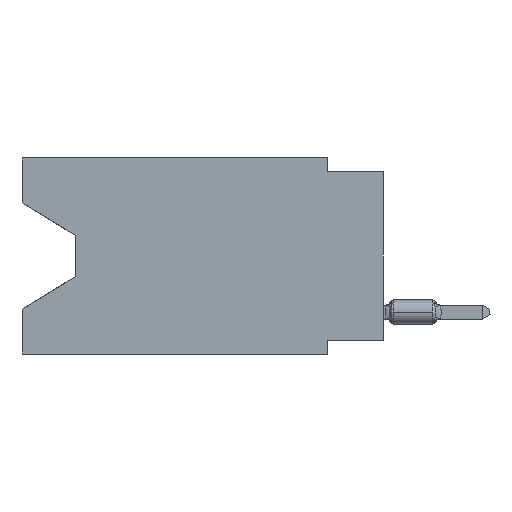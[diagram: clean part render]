
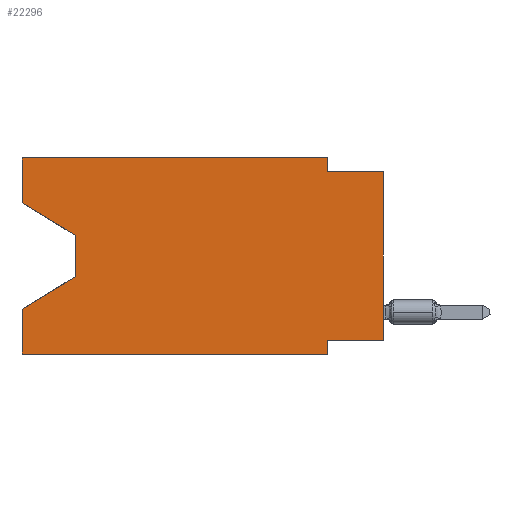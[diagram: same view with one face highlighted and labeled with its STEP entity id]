
A CAD part, left-side view. The second image highlights one B-rep face of the part: STEP entity #22296.
In plain terms, the highlighted planar face has unit normal (-1, 0, 0).
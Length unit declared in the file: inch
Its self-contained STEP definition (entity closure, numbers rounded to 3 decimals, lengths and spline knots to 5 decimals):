
#964 = CARTESIAN_POINT ( 'NONE',  ( 0., 0.645, 0. ) ) ;
#1428 = EDGE_CURVE ( 'NONE', #8827, #56739, #14687, .T. ) ;
#2313 = DIRECTION ( 'NONE',  ( 0., -1., 0. ) ) ;
#3526 = VERTEX_POINT ( 'NONE', #34012 ) ;
#4070 = CARTESIAN_POINT ( 'NONE',  ( 0., 0.55, -0.212 ) ) ;
#4557 = ORIENTED_EDGE ( 'NONE', *, *, #1428, .F. ) ;
#4574 = VERTEX_POINT ( 'NONE', #27284 ) ;
#5607 = VERTEX_POINT ( 'NONE', #44776 ) ;
#6593 = VECTOR ( 'NONE', #7825, 39.37008 ) ;
#6645 = DIRECTION ( 'NONE',  ( 0., 0., 1. ) ) ;
#7280 = CARTESIAN_POINT ( 'NONE',  ( 0., 0., -0.325 ) ) ;
#7825 = DIRECTION ( 'NONE',  ( 0., 0.855, -0.519 ) ) ;
#8555 = DIRECTION ( 'NONE',  ( 0., 0., 1. ) ) ;
#8827 = VERTEX_POINT ( 'NONE', #23724 ) ;
#10400 = EDGE_CURVE ( 'NONE', #5607, #15619, #30885, .T. ) ;
#10665 = LINE ( 'NONE', #19265, #46257 ) ;
#10930 = CARTESIAN_POINT ( 'NONE',  ( 0., 0.645, 0. ) ) ;
#11204 = FACE_OUTER_BOUND ( 'NONE', #55167, .T. ) ;
#11946 = ORIENTED_EDGE ( 'NONE', *, *, #47086, .F. ) ;
#12207 = CARTESIAN_POINT ( 'NONE',  ( 0., 0.645, -0.08025 ) ) ;
#12416 = VERTEX_POINT ( 'NONE', #50872 ) ;
#12481 = EDGE_CURVE ( 'NONE', #49396, #56739, #15259, .T. ) ;
#12950 = CARTESIAN_POINT ( 'NONE',  ( 0., 0.1, -0.35 ) ) ;
#13153 = LINE ( 'NONE', #21472, #21382 ) ;
#13313 = VECTOR ( 'NONE', #46690, 39.37008 ) ;
#13535 = CARTESIAN_POINT ( 'NONE',  ( 0., 0., -0.025 ) ) ;
#14687 = LINE ( 'NONE', #23007, #40045 ) ;
#15259 = LINE ( 'NONE', #29590, #23936 ) ;
#15532 = DIRECTION ( 'NONE',  ( 0., 0., -1. ) ) ;
#15619 = VERTEX_POINT ( 'NONE', #42896 ) ;
#15879 = VERTEX_POINT ( 'NONE', #16654 ) ;
#15883 = CARTESIAN_POINT ( 'NONE',  ( 0., 0.645, -0.26975 ) ) ;
#16369 = ORIENTED_EDGE ( 'NONE', *, *, #50506, .T. ) ;
#16379 = ORIENTED_EDGE ( 'NONE', *, *, #12481, .T. ) ;
#16654 = CARTESIAN_POINT ( 'NONE',  ( 0., 0.55, -0.212 ) ) ;
#16990 = LINE ( 'NONE', #46628, #45566 ) ;
#17529 = ORIENTED_EDGE ( 'NONE', *, *, #39760, .F. ) ;
#18486 = DIRECTION ( 'NONE',  ( 0., -1., 0. ) ) ;
#18595 = ORIENTED_EDGE ( 'NONE', *, *, #30845, .F. ) ;
#19265 = CARTESIAN_POINT ( 'NONE',  ( 0., 0.55, -0.138 ) ) ;
#20377 = CARTESIAN_POINT ( 'NONE',  ( 0., 0., -0.325 ) ) ;
#20718 = VERTEX_POINT ( 'NONE', #33764 ) ;
#21382 = VECTOR ( 'NONE', #8555, 39.37008 ) ;
#21472 = CARTESIAN_POINT ( 'NONE',  ( 0., 0.645, 0. ) ) ;
#21675 = AXIS2_PLACEMENT_3D ( 'NONE', #10930, #37353, #31905 ) ;
#21989 = EDGE_CURVE ( 'NONE', #12416, #55998, #16990, .T. ) ;
#22296 = ADVANCED_FACE ( 'NONE', ( #11204 ), #53731, .F. ) ;
#22534 = CARTESIAN_POINT ( 'NONE',  ( 0., 0.645, 0. ) ) ;
#23007 = CARTESIAN_POINT ( 'NONE',  ( 0., 0., -0.025 ) ) ;
#23724 = CARTESIAN_POINT ( 'NONE',  ( 0., 0.1, -0.025 ) ) ;
#23936 = VECTOR ( 'NONE', #6645, 39.37008 ) ;
#25617 = LINE ( 'NONE', #4070, #6593 ) ;
#27284 = CARTESIAN_POINT ( 'NONE',  ( 0., 0.55, -0.138 ) ) ;
#29590 = CARTESIAN_POINT ( 'NONE',  ( 0., 0., 0. ) ) ;
#29688 = DIRECTION ( 'NONE',  ( 0., 0., -1. ) ) ;
#30845 = EDGE_CURVE ( 'NONE', #20718, #55998, #56139, .T. ) ;
#30885 = LINE ( 'NONE', #22534, #44142 ) ;
#31681 = ORIENTED_EDGE ( 'NONE', *, *, #21989, .T. ) ;
#31689 = ORIENTED_EDGE ( 'NONE', *, *, #42534, .T. ) ;
#31905 = DIRECTION ( 'NONE',  ( 0., 0., -1. ) ) ;
#32025 = ORIENTED_EDGE ( 'NONE', *, *, #36731, .T. ) ;
#33203 = VECTOR ( 'NONE', #29688, 39.37008 ) ;
#33396 = LINE ( 'NONE', #7280, #54492 ) ;
#33764 = CARTESIAN_POINT ( 'NONE',  ( 0., 0.1, -0.325 ) ) ;
#34012 = CARTESIAN_POINT ( 'NONE',  ( 0., 0.1, 0. ) ) ;
#34922 = DIRECTION ( 'NONE',  ( 0., 0., -1. ) ) ;
#36321 = DIRECTION ( 'NONE',  ( 0., 0., 1. ) ) ;
#36731 = EDGE_CURVE ( 'NONE', #15879, #44504, #25617, .T. ) ;
#37353 = DIRECTION ( 'NONE',  ( 1., 0., 0. ) ) ;
#37779 = ORIENTED_EDGE ( 'NONE', *, *, #50207, .F. ) ;
#38364 = LINE ( 'NONE', #12207, #13313 ) ;
#39760 = EDGE_CURVE ( 'NONE', #12416, #44504, #13153, .T. ) ;
#40045 = VECTOR ( 'NONE', #2313, 39.37008 ) ;
#40340 = LINE ( 'NONE', #964, #40371 ) ;
#40371 = VECTOR ( 'NONE', #18486, 39.37008 ) ;
#42534 = EDGE_CURVE ( 'NONE', #5607, #4574, #38364, .T. ) ;
#42896 = CARTESIAN_POINT ( 'NONE',  ( 0., 0.645, 0. ) ) ;
#42935 = CARTESIAN_POINT ( 'NONE',  ( 0., 0.1, -0.35 ) ) ;
#43850 = CARTESIAN_POINT ( 'NONE',  ( 0., 0.1, 0. ) ) ;
#44142 = VECTOR ( 'NONE', #36321, 39.37008 ) ;
#44504 = VERTEX_POINT ( 'NONE', #15883 ) ;
#44776 = CARTESIAN_POINT ( 'NONE',  ( 0., 0.645, -0.08025 ) ) ;
#45566 = VECTOR ( 'NONE', #52065, 39.37008 ) ;
#46257 = VECTOR ( 'NONE', #15532, 39.37008 ) ;
#46628 = CARTESIAN_POINT ( 'NONE',  ( 0., 0.645, -0.35 ) ) ;
#46690 = DIRECTION ( 'NONE',  ( 0., -0.855, -0.519 ) ) ;
#47086 = EDGE_CURVE ( 'NONE', #3526, #8827, #52729, .T. ) ;
#48827 = EDGE_CURVE ( 'NONE', #15619, #3526, #40340, .T. ) ;
#49396 = VERTEX_POINT ( 'NONE', #20377 ) ;
#49408 = VECTOR ( 'NONE', #34922, 39.37008 ) ;
#49904 = ORIENTED_EDGE ( 'NONE', *, *, #48827, .F. ) ;
#50207 = EDGE_CURVE ( 'NONE', #49396, #20718, #33396, .T. ) ;
#50506 = EDGE_CURVE ( 'NONE', #4574, #15879, #10665, .T. ) ;
#50872 = CARTESIAN_POINT ( 'NONE',  ( 0., 0.645, -0.35 ) ) ;
#52065 = DIRECTION ( 'NONE',  ( 0., -1., 0. ) ) ;
#52729 = LINE ( 'NONE', #43850, #49408 ) ;
#53731 = PLANE ( 'NONE',  #21675 ) ;
#54492 = VECTOR ( 'NONE', #55821, 39.37008 ) ;
#55167 = EDGE_LOOP ( 'NONE', ( #31689, #16369, #32025, #17529, #31681, #18595, #37779, #16379, #4557, #11946, #49904, #56365 ) ) ;
#55821 = DIRECTION ( 'NONE',  ( 0., 1., 0. ) ) ;
#55998 = VERTEX_POINT ( 'NONE', #12950 ) ;
#56139 = LINE ( 'NONE', #42935, #33203 ) ;
#56365 = ORIENTED_EDGE ( 'NONE', *, *, #10400, .F. ) ;
#56739 = VERTEX_POINT ( 'NONE', #13535 ) ;
